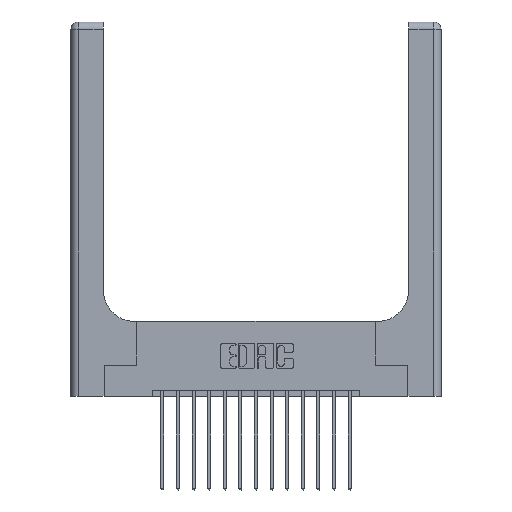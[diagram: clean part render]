
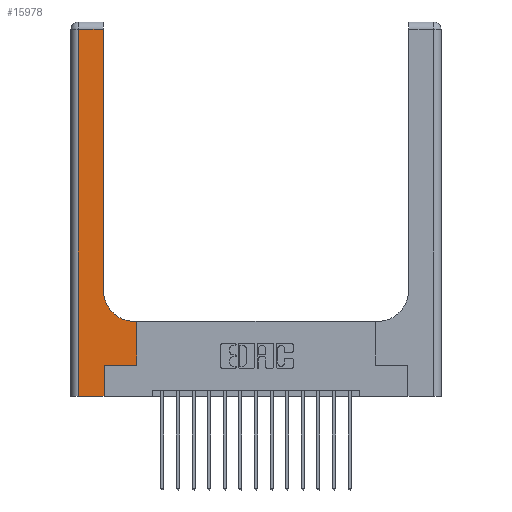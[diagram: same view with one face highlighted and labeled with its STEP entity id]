
A CAD part, top view. The second image highlights one B-rep face of the part: STEP entity #15978.
In plain terms, the highlighted planar face has unit normal (0, 0, 1).
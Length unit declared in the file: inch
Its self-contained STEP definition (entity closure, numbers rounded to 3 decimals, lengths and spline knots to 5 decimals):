
#121 = DIRECTION ( 'NONE',  ( 1., 0., 0. ) ) ;
#438 = CARTESIAN_POINT ( 'NONE',  ( 0., 2.94, 0.37 ) ) ;
#780 = VERTEX_POINT ( 'NONE', #10978 ) ;
#1017 = CARTESIAN_POINT ( 'NONE',  ( 0.26, 3., 0.37 ) ) ;
#1061 = CARTESIAN_POINT ( 'NONE',  ( 0.06, 0., 0.37 ) ) ;
#1349 = ORIENTED_EDGE ( 'NONE', *, *, #15859, .T. ) ;
#1450 = EDGE_CURVE ( 'NONE', #1918, #14368, #6369, .T. ) ;
#1601 = EDGE_CURVE ( 'NONE', #17518, #10571, #15213, .T. ) ;
#1792 = CARTESIAN_POINT ( 'NONE',  ( 0.528, 0.25, 0.37 ) ) ;
#1837 = CARTESIAN_POINT ( 'NONE',  ( 0.51, 0.6, 0.37 ) ) ;
#1889 = EDGE_LOOP ( 'NONE', ( #15732, #4356, #13802, #11090, #10123, #6812, #16728, #1349, #9125 ) ) ;
#1918 = VERTEX_POINT ( 'NONE', #17119 ) ;
#2489 = CARTESIAN_POINT ( 'NONE',  ( 0.528, 0.6, 0.37 ) ) ;
#2637 = DIRECTION ( 'NONE',  ( 0., 0., -1. ) ) ;
#2936 = VECTOR ( 'NONE', #121, 39.37008 ) ;
#2990 = VERTEX_POINT ( 'NONE', #2489 ) ;
#3260 = EDGE_CURVE ( 'NONE', #14368, #780, #15340, .T. ) ;
#3289 = CARTESIAN_POINT ( 'NONE',  ( 0.26, 0.6, 0.37 ) ) ;
#3368 = VECTOR ( 'NONE', #11290, 39.37008 ) ;
#3552 = AXIS2_PLACEMENT_3D ( 'NONE', #7744, #8846, #15965 ) ;
#4356 = ORIENTED_EDGE ( 'NONE', *, *, #5527, .T. ) ;
#4481 = DIRECTION ( 'NONE',  ( 1., 0., 0. ) ) ;
#4641 = EDGE_CURVE ( 'NONE', #11955, #1918, #11674, .T. ) ;
#5527 = EDGE_CURVE ( 'NONE', #10571, #13658, #10075, .T. ) ;
#5943 = CARTESIAN_POINT ( 'NONE',  ( 0., 0., 0.37 ) ) ;
#6369 = LINE ( 'NONE', #13389, #11611 ) ;
#6460 = DIRECTION ( 'NONE',  ( 0., 1., 0. ) ) ;
#6812 = ORIENTED_EDGE ( 'NONE', *, *, #3260, .T. ) ;
#6903 = PLANE ( 'NONE',  #15484 ) ;
#7017 = CARTESIAN_POINT ( 'NONE',  ( 0.06, 3., 0.37 ) ) ;
#7162 = DIRECTION ( 'NONE',  ( -1., 0., 0. ) ) ;
#7528 = VECTOR ( 'NONE', #13854, 39.37008 ) ;
#7744 = CARTESIAN_POINT ( 'NONE',  ( 0.51, 0.85, 0.37 ) ) ;
#8288 = CARTESIAN_POINT ( 'NONE',  ( 0., 3., 0.37 ) ) ;
#8439 = EDGE_CURVE ( 'NONE', #780, #2990, #14798, .T. ) ;
#8485 = VECTOR ( 'NONE', #4481, 39.37008 ) ;
#8826 = VECTOR ( 'NONE', #14185, 39.37008 ) ;
#8846 = DIRECTION ( 'NONE',  ( 0., 0., -1. ) ) ;
#9125 = ORIENTED_EDGE ( 'NONE', *, *, #15884, .T. ) ;
#10075 = LINE ( 'NONE', #438, #10535 ) ;
#10123 = ORIENTED_EDGE ( 'NONE', *, *, #1450, .T. ) ;
#10535 = VECTOR ( 'NONE', #7162, 39.37008 ) ;
#10571 = VERTEX_POINT ( 'NONE', #10832 ) ;
#10832 = CARTESIAN_POINT ( 'NONE',  ( 0.26, 2.94, 0.37 ) ) ;
#10978 = CARTESIAN_POINT ( 'NONE',  ( 0.528, 0.25, 0.37 ) ) ;
#11090 = ORIENTED_EDGE ( 'NONE', *, *, #4641, .T. ) ;
#11143 = EDGE_CURVE ( 'NONE', #13658, #11955, #16614, .T. ) ;
#11290 = DIRECTION ( 'NONE',  ( 0., -1., 0. ) ) ;
#11392 = CIRCLE ( 'NONE', #3552, 0.25 ) ;
#11611 = VECTOR ( 'NONE', #6460, 39.37008 ) ;
#11674 = LINE ( 'NONE', #5943, #8485 ) ;
#11955 = VERTEX_POINT ( 'NONE', #1061 ) ;
#12175 = CARTESIAN_POINT ( 'NONE',  ( 0.265, 0.25, 0.37 ) ) ;
#12587 = CARTESIAN_POINT ( 'NONE',  ( 0.265, 0.25, 0.37 ) ) ;
#13389 = CARTESIAN_POINT ( 'NONE',  ( 0.265, 0., 0.37 ) ) ;
#13658 = VERTEX_POINT ( 'NONE', #14320 ) ;
#13668 = FACE_OUTER_BOUND ( 'NONE', #1889, .T. ) ;
#13684 = VERTEX_POINT ( 'NONE', #1837 ) ;
#13802 = ORIENTED_EDGE ( 'NONE', *, *, #11143, .T. ) ;
#13854 = DIRECTION ( 'NONE',  ( 0., 1., 0. ) ) ;
#14034 = VECTOR ( 'NONE', #17506, 39.37008 ) ;
#14185 = DIRECTION ( 'NONE',  ( 0., 1., 0. ) ) ;
#14320 = CARTESIAN_POINT ( 'NONE',  ( 0.06, 2.94, 0.37 ) ) ;
#14368 = VERTEX_POINT ( 'NONE', #12175 ) ;
#14585 = LINE ( 'NONE', #3289, #14034 ) ;
#14798 = LINE ( 'NONE', #1792, #8826 ) ;
#15213 = LINE ( 'NONE', #1017, #7528 ) ;
#15340 = LINE ( 'NONE', #12587, #2936 ) ;
#15484 = AXIS2_PLACEMENT_3D ( 'NONE', #8288, #2637, #16239 ) ;
#15732 = ORIENTED_EDGE ( 'NONE', *, *, #1601, .T. ) ;
#15859 = EDGE_CURVE ( 'NONE', #2990, #13684, #14585, .T. ) ;
#15884 = EDGE_CURVE ( 'NONE', #13684, #17518, #11392, .T. ) ;
#15965 = DIRECTION ( 'NONE',  ( 1., 0., 0. ) ) ;
#15978 = ADVANCED_FACE ( 'NONE', ( #13668 ), #6903, .F. ) ;
#16239 = DIRECTION ( 'NONE',  ( -1., 0., 0. ) ) ;
#16614 = LINE ( 'NONE', #7017, #3368 ) ;
#16728 = ORIENTED_EDGE ( 'NONE', *, *, #8439, .T. ) ;
#17119 = CARTESIAN_POINT ( 'NONE',  ( 0.265, 0., 0.37 ) ) ;
#17484 = CARTESIAN_POINT ( 'NONE',  ( 0.26, 0.85, 0.37 ) ) ;
#17506 = DIRECTION ( 'NONE',  ( -1., 0., 0. ) ) ;
#17518 = VERTEX_POINT ( 'NONE', #17484 ) ;
